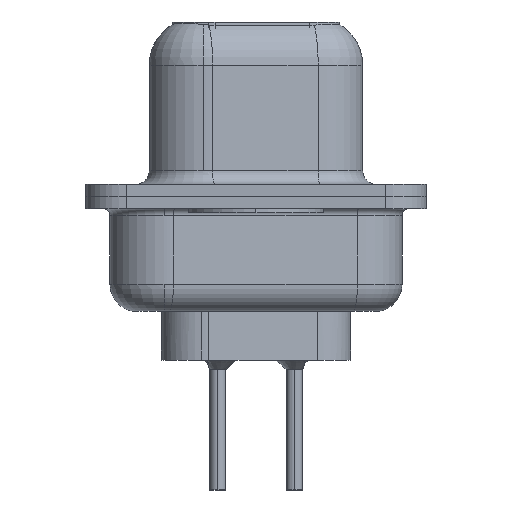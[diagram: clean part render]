
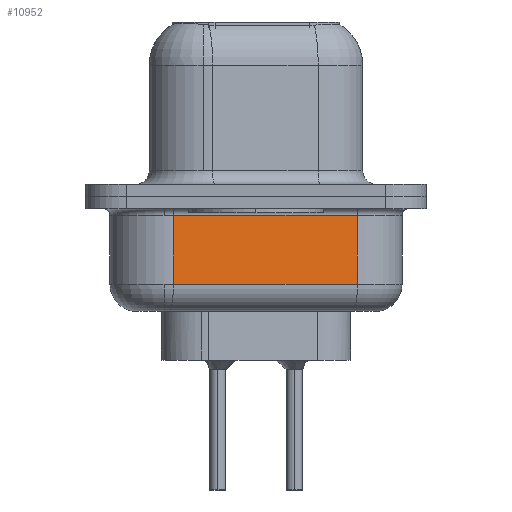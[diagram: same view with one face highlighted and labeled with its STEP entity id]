
A CAD part, left-side view. The second image highlights one B-rep face of the part: STEP entity #10952.
In plain terms, the highlighted planar face has unit normal (-0.985, -0.174, 0).
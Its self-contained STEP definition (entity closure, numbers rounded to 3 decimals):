
#967 = VERTEX_POINT ( 'NONE', #8729 ) ;
#2034 = CARTESIAN_POINT ( 'NONE',  ( 2.89, 3.053, -4.25 ) ) ;
#2856 = VECTOR ( 'NONE', #21641, 1000. ) ;
#3173 = VECTOR ( 'NONE', #11103, 1000. ) ;
#3883 = CARTESIAN_POINT ( 'NONE',  ( 2.89, 3.053, -4.25 ) ) ;
#4030 = EDGE_CURVE ( 'NONE', #18344, #14225, #20870, .T. ) ;
#5824 = EDGE_CURVE ( 'NONE', #11777, #967, #13009, .T. ) ;
#5852 = CARTESIAN_POINT ( 'NONE',  ( 4.089, -3.747, -4.25 ) ) ;
#5919 = DIRECTION ( 'NONE',  ( -0.174, 0.985, 0. ) ) ;
#6144 = FACE_OUTER_BOUND ( 'NONE', #8535, .T. ) ;
#7099 = EDGE_CURVE ( 'NONE', #18344, #11777, #16366, .T. ) ;
#8062 = ORIENTED_EDGE ( 'NONE', *, *, #7099, .T. ) ;
#8228 = ORIENTED_EDGE ( 'NONE', *, *, #4030, .F. ) ;
#8535 = EDGE_LOOP ( 'NONE', ( #8228, #8062, #18359, #11237 ) ) ;
#8729 = CARTESIAN_POINT ( 'NONE',  ( 4.089, -3.747, -0.7 ) ) ;
#8933 = LINE ( 'NONE', #12554, #14286 ) ;
#9731 = CARTESIAN_POINT ( 'NONE',  ( 2.89, 3.053, -3.25 ) ) ;
#10952 = ADVANCED_FACE ( 'NONE', ( #6144 ), #21608, .F. ) ;
#11103 = DIRECTION ( 'NONE',  ( 0.174, -0.985, 0. ) ) ;
#11237 = ORIENTED_EDGE ( 'NONE', *, *, #18473, .T. ) ;
#11777 = VERTEX_POINT ( 'NONE', #17824 ) ;
#12554 = CARTESIAN_POINT ( 'NONE',  ( 2.89, 3.053, -0.7 ) ) ;
#13009 = LINE ( 'NONE', #5852, #2856 ) ;
#14225 = VERTEX_POINT ( 'NONE', #20132 ) ;
#14286 = VECTOR ( 'NONE', #19380, 1000. ) ;
#14770 = DIRECTION ( 'NONE',  ( 0.985, 0.174, 0. ) ) ;
#15039 = CARTESIAN_POINT ( 'NONE',  ( 2.89, 3.053, -3.25 ) ) ;
#16366 = LINE ( 'NONE', #9731, #3173 ) ;
#17633 = VECTOR ( 'NONE', #19068, 1000. ) ;
#17824 = CARTESIAN_POINT ( 'NONE',  ( 4.089, -3.747, -3.25 ) ) ;
#18344 = VERTEX_POINT ( 'NONE', #15039 ) ;
#18359 = ORIENTED_EDGE ( 'NONE', *, *, #5824, .T. ) ;
#18473 = EDGE_CURVE ( 'NONE', #967, #14225, #8933, .T. ) ;
#19068 = DIRECTION ( 'NONE',  ( 0., 0., 1. ) ) ;
#19380 = DIRECTION ( 'NONE',  ( -0.174, 0.985, 0. ) ) ;
#20132 = CARTESIAN_POINT ( 'NONE',  ( 2.89, 3.053, -0.7 ) ) ;
#20144 = AXIS2_PLACEMENT_3D ( 'NONE', #3883, #14770, #5919 ) ;
#20870 = LINE ( 'NONE', #2034, #17633 ) ;
#21608 = PLANE ( 'NONE',  #20144 ) ;
#21641 = DIRECTION ( 'NONE',  ( 0., 0., 1. ) ) ;
